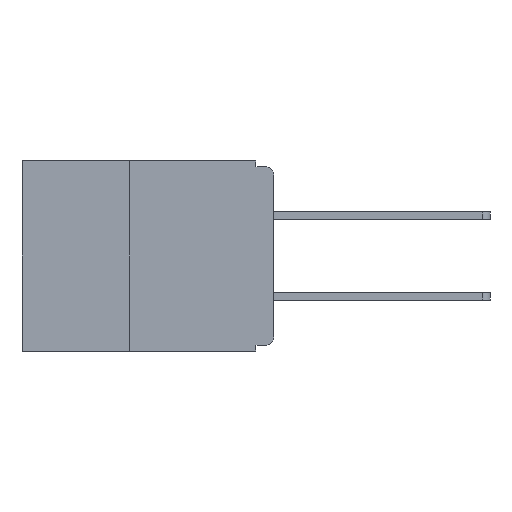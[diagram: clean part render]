
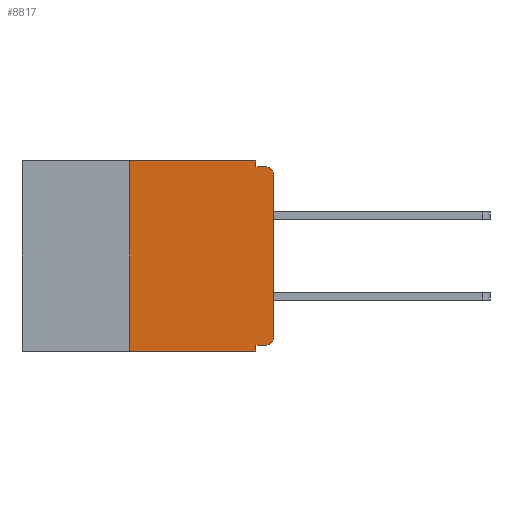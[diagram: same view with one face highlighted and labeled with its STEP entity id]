
A CAD part, left-side view. The second image highlights one B-rep face of the part: STEP entity #8817.
In plain terms, the highlighted planar face has unit normal (-1, 0, 0).
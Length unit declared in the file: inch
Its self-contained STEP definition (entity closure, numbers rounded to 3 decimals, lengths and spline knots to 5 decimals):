
#695 = DIRECTION ( 'NONE',  ( 0., 0., 1. ) ) ;
#994 = VECTOR ( 'NONE', #16307, 39.37008 ) ;
#1039 = CARTESIAN_POINT ( 'NONE',  ( 0., 0.437, -0.33 ) ) ;
#1585 = ORIENTED_EDGE ( 'NONE', *, *, #19208, .T. ) ;
#1762 = DIRECTION ( 'NONE',  ( 1., 0., 0. ) ) ;
#2204 = EDGE_CURVE ( 'NONE', #15106, #16590, #18943, .T. ) ;
#2764 = CARTESIAN_POINT ( 'NONE',  ( 0., 0.015, -0.32 ) ) ;
#2902 = EDGE_CURVE ( 'NONE', #9427, #3354, #24944, .T. ) ;
#3354 = VERTEX_POINT ( 'NONE', #28136 ) ;
#3806 = ORIENTED_EDGE ( 'NONE', *, *, #21978, .F. ) ;
#3892 = EDGE_CURVE ( 'NONE', #7564, #3354, #9674, .T. ) ;
#4797 = ORIENTED_EDGE ( 'NONE', *, *, #9834, .F. ) ;
#5063 = LINE ( 'NONE', #15307, #18834 ) ;
#5946 = VECTOR ( 'NONE', #24437, 39.37008 ) ;
#6684 = EDGE_LOOP ( 'NONE', ( #30181, #20147, #3806, #9504, #14586, #4797, #31002, #12105, #16486, #1585 ) ) ;
#7388 = CARTESIAN_POINT ( 'NONE',  ( 0., 0., -0.01 ) ) ;
#7485 = VERTEX_POINT ( 'NONE', #10578 ) ;
#7488 = EDGE_CURVE ( 'NONE', #14751, #9427, #9104, .T. ) ;
#7564 = VERTEX_POINT ( 'NONE', #13314 ) ;
#8817 = ADVANCED_FACE ( 'NONE', ( #9011 ), #13985, .F. ) ;
#9011 = FACE_OUTER_BOUND ( 'NONE', #6684, .T. ) ;
#9104 = LINE ( 'NONE', #13000, #14795 ) ;
#9427 = VERTEX_POINT ( 'NONE', #28266 ) ;
#9504 = ORIENTED_EDGE ( 'NONE', *, *, #20695, .F. ) ;
#9674 = LINE ( 'NONE', #1039, #21091 ) ;
#9718 = VERTEX_POINT ( 'NONE', #14861 ) ;
#9834 = EDGE_CURVE ( 'NONE', #7564, #22974, #17276, .T. ) ;
#10578 = CARTESIAN_POINT ( 'NONE',  ( 0., 0., -0.305 ) ) ;
#10750 = CIRCLE ( 'NONE', #22354, 0.015 ) ;
#10793 = CARTESIAN_POINT ( 'NONE',  ( 0., 0.031, -0.01 ) ) ;
#10972 = EDGE_CURVE ( 'NONE', #7485, #15106, #5063, .T. ) ;
#12026 = VECTOR ( 'NONE', #28909, 39.37008 ) ;
#12105 = ORIENTED_EDGE ( 'NONE', *, *, #2902, .F. ) ;
#12849 = CARTESIAN_POINT ( 'NONE',  ( 0., 0.25, -0.33 ) ) ;
#13000 = CARTESIAN_POINT ( 'NONE',  ( 0., 0., -0.32 ) ) ;
#13076 = DIRECTION ( 'NONE',  ( -1., 0., 0. ) ) ;
#13314 = CARTESIAN_POINT ( 'NONE',  ( 0., 0.25, -0.33 ) ) ;
#13985 = PLANE ( 'NONE',  #27370 ) ;
#14014 = LINE ( 'NONE', #23705, #994 ) ;
#14285 = DIRECTION ( 'NONE',  ( 0., 0., -1. ) ) ;
#14586 = ORIENTED_EDGE ( 'NONE', *, *, #28205, .F. ) ;
#14751 = VERTEX_POINT ( 'NONE', #2764 ) ;
#14795 = VECTOR ( 'NONE', #29989, 39.37008 ) ;
#14861 = CARTESIAN_POINT ( 'NONE',  ( 0., 0.031, 0. ) ) ;
#14943 = CARTESIAN_POINT ( 'NONE',  ( 0., 0.015, -0.01 ) ) ;
#15106 = VERTEX_POINT ( 'NONE', #16184 ) ;
#15307 = CARTESIAN_POINT ( 'NONE',  ( 0., 0., 0. ) ) ;
#16184 = CARTESIAN_POINT ( 'NONE',  ( 0., 0., -0.025 ) ) ;
#16307 = DIRECTION ( 'NONE',  ( 0., -1., 0. ) ) ;
#16486 = ORIENTED_EDGE ( 'NONE', *, *, #7488, .F. ) ;
#16590 = VERTEX_POINT ( 'NONE', #14943 ) ;
#16607 = CARTESIAN_POINT ( 'NONE',  ( 0., 0.031, 0. ) ) ;
#16705 = VECTOR ( 'NONE', #14285, 39.37008 ) ;
#17276 = LINE ( 'NONE', #12849, #24542 ) ;
#18834 = VECTOR ( 'NONE', #695, 39.37008 ) ;
#18896 = DIRECTION ( 'NONE',  ( 0., 0., -1. ) ) ;
#18943 = CIRCLE ( 'NONE', #23211, 0.015 ) ;
#19182 = CARTESIAN_POINT ( 'NONE',  ( 0., 0.031, -0.33 ) ) ;
#19208 = EDGE_CURVE ( 'NONE', #14751, #7485, #10750, .T. ) ;
#20147 = ORIENTED_EDGE ( 'NONE', *, *, #2204, .T. ) ;
#20591 = DIRECTION ( 'NONE',  ( 0., -1., 0. ) ) ;
#20695 = EDGE_CURVE ( 'NONE', #9718, #29558, #30393, .T. ) ;
#21091 = VECTOR ( 'NONE', #20591, 39.37008 ) ;
#21978 = EDGE_CURVE ( 'NONE', #29558, #16590, #23908, .T. ) ;
#22354 = AXIS2_PLACEMENT_3D ( 'NONE', #27642, #13076, #30065 ) ;
#22974 = VERTEX_POINT ( 'NONE', #23216 ) ;
#23211 = AXIS2_PLACEMENT_3D ( 'NONE', #29987, #31506, #26318 ) ;
#23216 = CARTESIAN_POINT ( 'NONE',  ( 0., 0.25, 0. ) ) ;
#23705 = CARTESIAN_POINT ( 'NONE',  ( 0., 0.437, 0. ) ) ;
#23908 = LINE ( 'NONE', #7388, #5946 ) ;
#24437 = DIRECTION ( 'NONE',  ( 0., -1., 0. ) ) ;
#24542 = VECTOR ( 'NONE', #29822, 39.37008 ) ;
#24944 = LINE ( 'NONE', #19182, #12026 ) ;
#26318 = DIRECTION ( 'NONE',  ( 0., 0., -1. ) ) ;
#27370 = AXIS2_PLACEMENT_3D ( 'NONE', #30945, #1762, #18896 ) ;
#27642 = CARTESIAN_POINT ( 'NONE',  ( 0., 0.015, -0.305 ) ) ;
#28136 = CARTESIAN_POINT ( 'NONE',  ( 0., 0.031, -0.33 ) ) ;
#28205 = EDGE_CURVE ( 'NONE', #22974, #9718, #14014, .T. ) ;
#28266 = CARTESIAN_POINT ( 'NONE',  ( 0., 0.031, -0.32 ) ) ;
#28909 = DIRECTION ( 'NONE',  ( 0., 0., -1. ) ) ;
#29558 = VERTEX_POINT ( 'NONE', #10793 ) ;
#29822 = DIRECTION ( 'NONE',  ( 0., 0., 1. ) ) ;
#29987 = CARTESIAN_POINT ( 'NONE',  ( 0., 0.015, -0.025 ) ) ;
#29989 = DIRECTION ( 'NONE',  ( 0., 1., 0. ) ) ;
#30065 = DIRECTION ( 'NONE',  ( 0., 0., -1. ) ) ;
#30181 = ORIENTED_EDGE ( 'NONE', *, *, #10972, .T. ) ;
#30393 = LINE ( 'NONE', #16607, #16705 ) ;
#30945 = CARTESIAN_POINT ( 'NONE',  ( 0., 0.437, 0. ) ) ;
#31002 = ORIENTED_EDGE ( 'NONE', *, *, #3892, .T. ) ;
#31506 = DIRECTION ( 'NONE',  ( -1., 0., 0. ) ) ;
